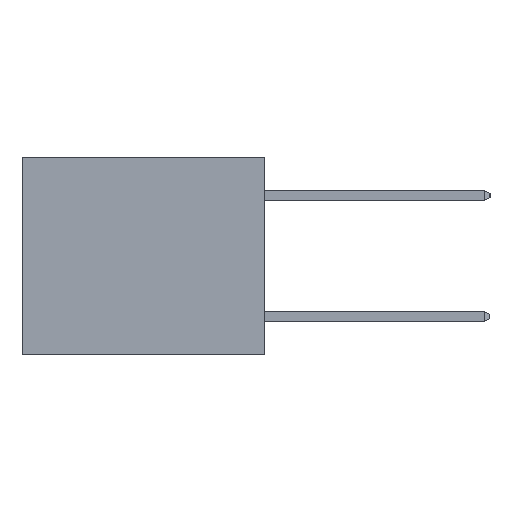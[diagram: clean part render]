
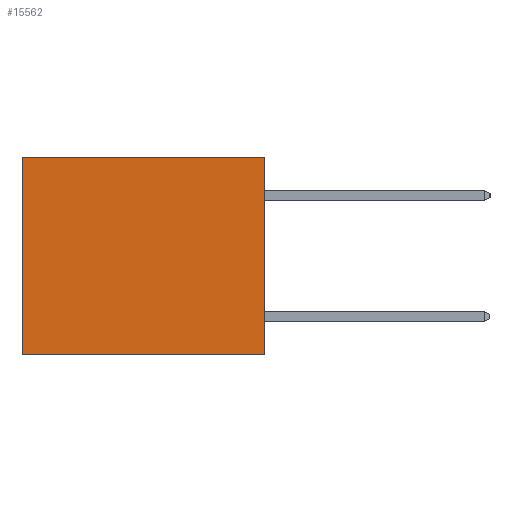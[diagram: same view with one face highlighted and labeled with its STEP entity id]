
A CAD part, left-side view. The second image highlights one B-rep face of the part: STEP entity #15562.
In plain terms, the highlighted planar face has unit normal (-1, 0, 0).
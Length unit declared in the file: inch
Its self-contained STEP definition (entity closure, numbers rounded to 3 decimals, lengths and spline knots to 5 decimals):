
#262 = DIRECTION ( 'NONE',  ( 0., 1., 0. ) ) ;
#801 = EDGE_LOOP ( 'NONE', ( #3064, #8970, #8677, #18960 ) ) ;
#1142 = DIRECTION ( 'NONE',  ( 1., 0., 0. ) ) ;
#1582 = VERTEX_POINT ( 'NONE', #9779 ) ;
#3064 = ORIENTED_EDGE ( 'NONE', *, *, #11992, .T. ) ;
#4121 = LINE ( 'NONE', #9438, #18371 ) ;
#4681 = CARTESIAN_POINT ( 'NONE',  ( 0.3165, 0.6, -0.49 ) ) ;
#4859 = VECTOR ( 'NONE', #7116, 39.37008 ) ;
#4895 = EDGE_CURVE ( 'NONE', #16348, #1582, #5305, .T. ) ;
#4927 = VERTEX_POINT ( 'NONE', #14771 ) ;
#5289 = DIRECTION ( 'NONE',  ( 0., 1., 0. ) ) ;
#5305 = LINE ( 'NONE', #15933, #9422 ) ;
#6666 = AXIS2_PLACEMENT_3D ( 'NONE', #15774, #1142, #11396 ) ;
#7116 = DIRECTION ( 'NONE',  ( 0., 0., -1. ) ) ;
#7181 = CARTESIAN_POINT ( 'NONE',  ( 0.3165, 0.6, -0.49 ) ) ;
#7224 = EDGE_CURVE ( 'NONE', #4927, #17271, #4121, .T. ) ;
#7249 = CARTESIAN_POINT ( 'NONE',  ( 0.3165, 0., 0. ) ) ;
#7498 = FACE_OUTER_BOUND ( 'NONE', #801, .T. ) ;
#8677 = ORIENTED_EDGE ( 'NONE', *, *, #14435, .F. ) ;
#8970 = ORIENTED_EDGE ( 'NONE', *, *, #7224, .F. ) ;
#9422 = VECTOR ( 'NONE', #262, 39.37008 ) ;
#9438 = CARTESIAN_POINT ( 'NONE',  ( 0.3165, 0., -0.49 ) ) ;
#9779 = CARTESIAN_POINT ( 'NONE',  ( 0.3165, 0.6, 0. ) ) ;
#11396 = DIRECTION ( 'NONE',  ( 0., 0., -1. ) ) ;
#11992 = EDGE_CURVE ( 'NONE', #1582, #17271, #12159, .T. ) ;
#12159 = LINE ( 'NONE', #7181, #4859 ) ;
#12739 = PLANE ( 'NONE',  #6666 ) ;
#14006 = VECTOR ( 'NONE', #14541, 39.37008 ) ;
#14435 = EDGE_CURVE ( 'NONE', #16348, #4927, #17012, .T. ) ;
#14541 = DIRECTION ( 'NONE',  ( 0., 0., -1. ) ) ;
#14771 = CARTESIAN_POINT ( 'NONE',  ( 0.3165, 0., -0.49 ) ) ;
#15562 = ADVANCED_FACE ( 'NONE', ( #7498 ), #12739, .F. ) ;
#15774 = CARTESIAN_POINT ( 'NONE',  ( 0.3165, 0., -0.49 ) ) ;
#15933 = CARTESIAN_POINT ( 'NONE',  ( 0.3165, 0., 0. ) ) ;
#16035 = CARTESIAN_POINT ( 'NONE',  ( 0.3165, 0., -0.49 ) ) ;
#16348 = VERTEX_POINT ( 'NONE', #7249 ) ;
#17012 = LINE ( 'NONE', #16035, #14006 ) ;
#17271 = VERTEX_POINT ( 'NONE', #4681 ) ;
#18371 = VECTOR ( 'NONE', #5289, 39.37008 ) ;
#18960 = ORIENTED_EDGE ( 'NONE', *, *, #4895, .T. ) ;
